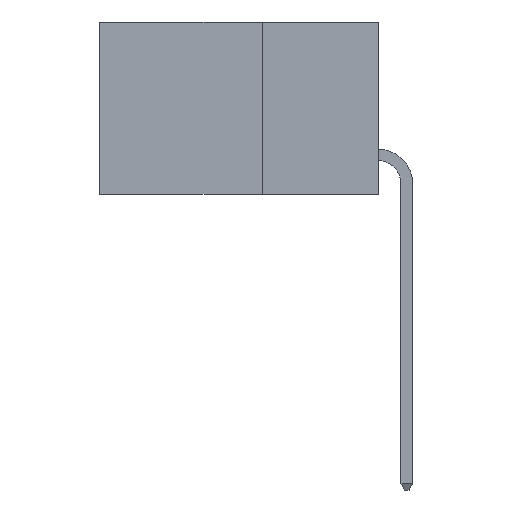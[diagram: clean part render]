
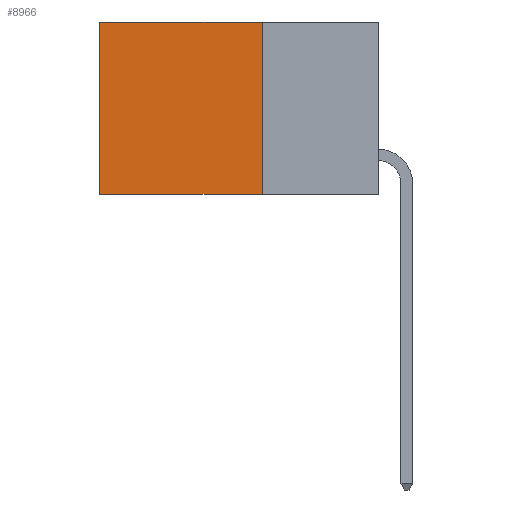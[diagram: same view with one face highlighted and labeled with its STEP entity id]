
A CAD part, left-side view. The second image highlights one B-rep face of the part: STEP entity #8966.
In plain terms, the highlighted planar face has unit normal (-1, 0, 0).
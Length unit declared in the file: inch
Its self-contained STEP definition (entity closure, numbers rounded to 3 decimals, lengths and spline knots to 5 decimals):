
#312 = VECTOR ( 'NONE', #2747, 39.37008 ) ;
#478 = DIRECTION ( 'NONE',  ( 1., 0., 0. ) ) ;
#524 = VERTEX_POINT ( 'NONE', #6851 ) ;
#711 = CARTESIAN_POINT ( 'NONE',  ( 0.2615, 0.6, -0.37 ) ) ;
#939 = EDGE_CURVE ( 'NONE', #12344, #524, #4226, .T. ) ;
#1511 = VECTOR ( 'NONE', #8033, 39.37008 ) ;
#1738 = CARTESIAN_POINT ( 'NONE',  ( 0.2615, 0.25, 0. ) ) ;
#1751 = CARTESIAN_POINT ( 'NONE',  ( 0.2615, 0.25, -0.37 ) ) ;
#2131 = CARTESIAN_POINT ( 'NONE',  ( 0.2615, 0.25, -0.37 ) ) ;
#2332 = CARTESIAN_POINT ( 'NONE',  ( 0.2615, 0.6, -0.37 ) ) ;
#2608 = LINE ( 'NONE', #1751, #312 ) ;
#2747 = DIRECTION ( 'NONE',  ( 0., 0., -1. ) ) ;
#2873 = VERTEX_POINT ( 'NONE', #2131 ) ;
#3294 = LINE ( 'NONE', #2332, #6216 ) ;
#3608 = EDGE_CURVE ( 'NONE', #2873, #7831, #9273, .T. ) ;
#3974 = EDGE_CURVE ( 'NONE', #12344, #2873, #2608, .T. ) ;
#4226 = LINE ( 'NONE', #6047, #9048 ) ;
#4966 = EDGE_CURVE ( 'NONE', #524, #7831, #3294, .T. ) ;
#5355 = FACE_OUTER_BOUND ( 'NONE', #10297, .T. ) ;
#6047 = CARTESIAN_POINT ( 'NONE',  ( 0.2615, 0.25, 0. ) ) ;
#6216 = VECTOR ( 'NONE', #9137, 39.37008 ) ;
#6365 = PLANE ( 'NONE',  #10146 ) ;
#6851 = CARTESIAN_POINT ( 'NONE',  ( 0.2615, 0.6, 0. ) ) ;
#7280 = ORIENTED_EDGE ( 'NONE', *, *, #4966, .T. ) ;
#7308 = DIRECTION ( 'NONE',  ( 0., 0., -1. ) ) ;
#7831 = VERTEX_POINT ( 'NONE', #711 ) ;
#8033 = DIRECTION ( 'NONE',  ( 0., 1., 0. ) ) ;
#8757 = DIRECTION ( 'NONE',  ( 0., 1., 0. ) ) ;
#8785 = ORIENTED_EDGE ( 'NONE', *, *, #939, .T. ) ;
#8871 = ORIENTED_EDGE ( 'NONE', *, *, #3974, .F. ) ;
#8966 = ADVANCED_FACE ( 'NONE', ( #5355 ), #6365, .F. ) ;
#9001 = CARTESIAN_POINT ( 'NONE',  ( 0.2615, 0.25, -0.37 ) ) ;
#9048 = VECTOR ( 'NONE', #8757, 39.37008 ) ;
#9137 = DIRECTION ( 'NONE',  ( 0., 0., -1. ) ) ;
#9273 = LINE ( 'NONE', #9001, #1511 ) ;
#9875 = ORIENTED_EDGE ( 'NONE', *, *, #3608, .F. ) ;
#10146 = AXIS2_PLACEMENT_3D ( 'NONE', #12035, #478, #7308 ) ;
#10297 = EDGE_LOOP ( 'NONE', ( #7280, #9875, #8871, #8785 ) ) ;
#12035 = CARTESIAN_POINT ( 'NONE',  ( 0.2615, 0.25, -0.37 ) ) ;
#12344 = VERTEX_POINT ( 'NONE', #1738 ) ;
